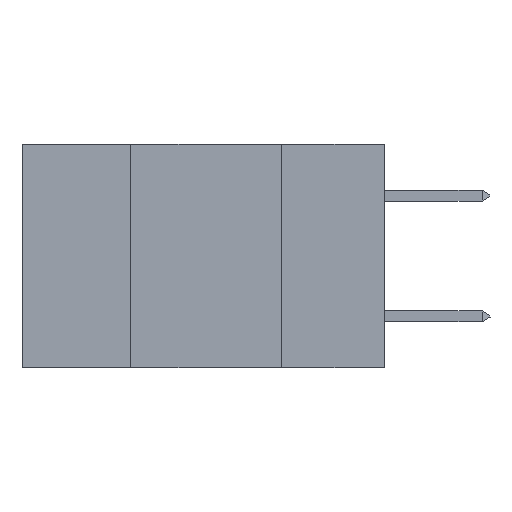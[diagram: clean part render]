
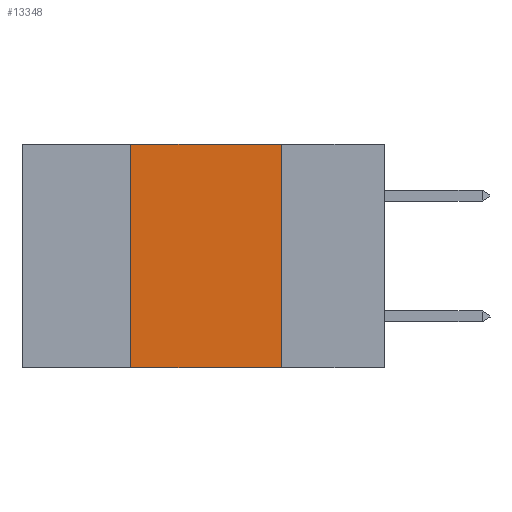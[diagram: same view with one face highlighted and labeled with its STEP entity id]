
A CAD part, left-side view. The second image highlights one B-rep face of the part: STEP entity #13348.
In plain terms, the highlighted planar face has unit normal (-1, 0, 0).
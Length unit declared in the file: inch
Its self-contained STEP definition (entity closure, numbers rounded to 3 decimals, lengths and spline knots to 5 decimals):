
#181 = PLANE ( 'NONE',  #9423 ) ;
#1136 = ORIENTED_EDGE ( 'NONE', *, *, #3717, .F. ) ;
#1699 = LINE ( 'NONE', #34331, #37374 ) ;
#2186 = DIRECTION ( 'NONE',  ( 0., -1., 0. ) ) ;
#3094 = CARTESIAN_POINT ( 'NONE',  ( 0., 0.6, 0. ) ) ;
#3717 = EDGE_CURVE ( 'NONE', #31995, #13374, #38013, .T. ) ;
#6102 = LINE ( 'NONE', #29175, #32376 ) ;
#6930 = CARTESIAN_POINT ( 'NONE',  ( 0., 0.42, 0. ) ) ;
#8206 = ORIENTED_EDGE ( 'NONE', *, *, #20218, .F. ) ;
#8542 = CARTESIAN_POINT ( 'NONE',  ( 0., 0.17, 0. ) ) ;
#9423 = AXIS2_PLACEMENT_3D ( 'NONE', #3094, #15846, #40904 ) ;
#9840 = DIRECTION ( 'NONE',  ( 0., -1., 0. ) ) ;
#13308 = EDGE_LOOP ( 'NONE', ( #8206, #1136, #24518, #14792 ) ) ;
#13341 = DIRECTION ( 'NONE',  ( 0., 0., 1. ) ) ;
#13348 = ADVANCED_FACE ( 'NONE', ( #36981 ), #181, .F. ) ;
#13374 = VERTEX_POINT ( 'NONE', #8542 ) ;
#14792 = ORIENTED_EDGE ( 'NONE', *, *, #31888, .T. ) ;
#15846 = DIRECTION ( 'NONE',  ( 1., 0., 0. ) ) ;
#16424 = CARTESIAN_POINT ( 'NONE',  ( 0., 0.42, 0. ) ) ;
#18835 = DIRECTION ( 'NONE',  ( 0., 0., -1. ) ) ;
#20218 = EDGE_CURVE ( 'NONE', #13374, #24116, #1699, .T. ) ;
#24116 = VERTEX_POINT ( 'NONE', #39841 ) ;
#24518 = ORIENTED_EDGE ( 'NONE', *, *, #27683, .F. ) ;
#26694 = CARTESIAN_POINT ( 'NONE',  ( 0., 0.42, -0.37 ) ) ;
#27595 = LINE ( 'NONE', #16424, #39075 ) ;
#27683 = EDGE_CURVE ( 'NONE', #34438, #31995, #27595, .T. ) ;
#29175 = CARTESIAN_POINT ( 'NONE',  ( 0., 0.6, -0.37 ) ) ;
#31888 = EDGE_CURVE ( 'NONE', #34438, #24116, #6102, .T. ) ;
#31995 = VERTEX_POINT ( 'NONE', #6930 ) ;
#32376 = VECTOR ( 'NONE', #9840, 39.37008 ) ;
#34331 = CARTESIAN_POINT ( 'NONE',  ( 0., 0.17, 0. ) ) ;
#34438 = VERTEX_POINT ( 'NONE', #26694 ) ;
#36563 = VECTOR ( 'NONE', #2186, 39.37008 ) ;
#36981 = FACE_OUTER_BOUND ( 'NONE', #13308, .T. ) ;
#37214 = CARTESIAN_POINT ( 'NONE',  ( 0., 0.6, 0. ) ) ;
#37374 = VECTOR ( 'NONE', #18835, 39.37008 ) ;
#38013 = LINE ( 'NONE', #37214, #36563 ) ;
#39075 = VECTOR ( 'NONE', #13341, 39.37008 ) ;
#39841 = CARTESIAN_POINT ( 'NONE',  ( 0., 0.17, -0.37 ) ) ;
#40904 = DIRECTION ( 'NONE',  ( 0., 0., -1. ) ) ;
